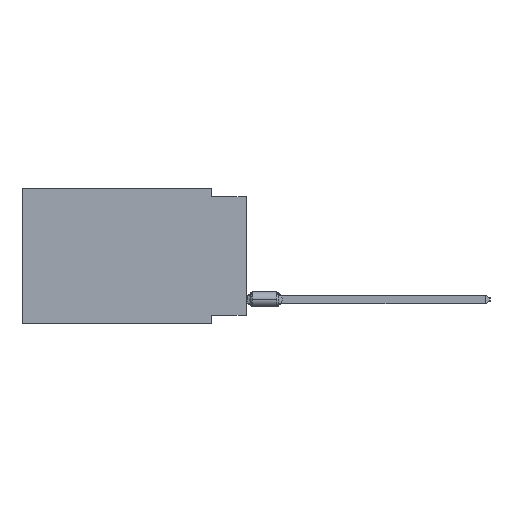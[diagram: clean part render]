
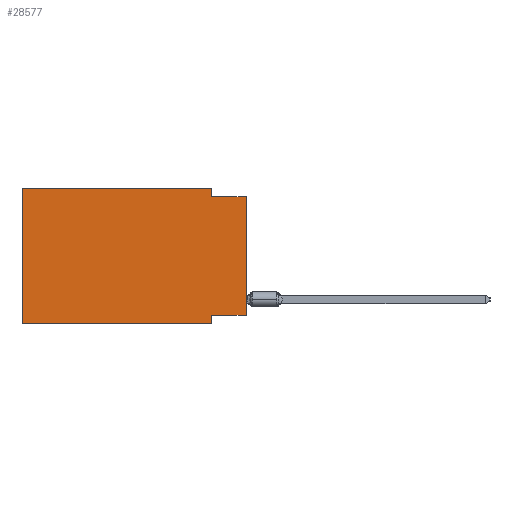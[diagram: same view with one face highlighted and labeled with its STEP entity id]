
A CAD part, left-side view. The second image highlights one B-rep face of the part: STEP entity #28577.
In plain terms, the highlighted planar face has unit normal (-1, 0, 0).
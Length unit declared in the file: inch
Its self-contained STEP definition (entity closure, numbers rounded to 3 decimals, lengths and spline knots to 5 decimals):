
#145 = VECTOR ( 'NONE', #30074, 39.37008 ) ;
#1103 = CARTESIAN_POINT ( 'NONE',  ( 0., 0., -0.365 ) ) ;
#1312 = DIRECTION ( 'NONE',  ( 0., -1., 0. ) ) ;
#1321 = ORIENTED_EDGE ( 'NONE', *, *, #29174, .T. ) ;
#2179 = CARTESIAN_POINT ( 'NONE',  ( 0., 0.645, 0. ) ) ;
#2435 = LINE ( 'NONE', #18656, #37084 ) ;
#2468 = LINE ( 'NONE', #34897, #15779 ) ;
#3201 = ORIENTED_EDGE ( 'NONE', *, *, #27384, .F. ) ;
#3221 = EDGE_CURVE ( 'NONE', #34792, #11804, #46527, .T. ) ;
#5310 = CARTESIAN_POINT ( 'NONE',  ( 0., 0.645, -0.39 ) ) ;
#5547 = CARTESIAN_POINT ( 'NONE',  ( 0., 0., -0.365 ) ) ;
#6477 = VECTOR ( 'NONE', #13910, 39.37008 ) ;
#7226 = DIRECTION ( 'NONE',  ( 0., 0., -1. ) ) ;
#8463 = ORIENTED_EDGE ( 'NONE', *, *, #50432, .F. ) ;
#8610 = VECTOR ( 'NONE', #34588, 39.37008 ) ;
#8622 = EDGE_CURVE ( 'NONE', #34792, #28995, #41442, .T. ) ;
#9359 = CARTESIAN_POINT ( 'NONE',  ( 0., 0.645, 0. ) ) ;
#11427 = CARTESIAN_POINT ( 'NONE',  ( 0., 0.1, 0. ) ) ;
#11472 = CARTESIAN_POINT ( 'NONE',  ( 0., 0., -0.025 ) ) ;
#11804 = VERTEX_POINT ( 'NONE', #32282 ) ;
#11856 = ORIENTED_EDGE ( 'NONE', *, *, #8622, .T. ) ;
#13594 = VERTEX_POINT ( 'NONE', #11427 ) ;
#13744 = VERTEX_POINT ( 'NONE', #33440 ) ;
#13910 = DIRECTION ( 'NONE',  ( 0., -1., 0. ) ) ;
#14241 = CARTESIAN_POINT ( 'NONE',  ( 0., 0.645, 0. ) ) ;
#14652 = EDGE_LOOP ( 'NONE', ( #1321, #3201, #19475, #15626, #17427, #11856, #8463, #35387 ) ) ;
#15626 = ORIENTED_EDGE ( 'NONE', *, *, #48692, .F. ) ;
#15779 = VECTOR ( 'NONE', #30926, 39.37008 ) ;
#16359 = VERTEX_POINT ( 'NONE', #1103 ) ;
#17427 = ORIENTED_EDGE ( 'NONE', *, *, #3221, .F. ) ;
#18045 = LINE ( 'NONE', #5547, #22637 ) ;
#18418 = LINE ( 'NONE', #22664, #6477 ) ;
#18656 = CARTESIAN_POINT ( 'NONE',  ( 0., 0.1, 0. ) ) ;
#19475 = ORIENTED_EDGE ( 'NONE', *, *, #33443, .F. ) ;
#21434 = VERTEX_POINT ( 'NONE', #30998 ) ;
#21688 = DIRECTION ( 'NONE',  ( 0., 0., -1. ) ) ;
#21935 = DIRECTION ( 'NONE',  ( 1., 0., 0. ) ) ;
#22637 = VECTOR ( 'NONE', #25992, 39.37008 ) ;
#22664 = CARTESIAN_POINT ( 'NONE',  ( 0., 0., -0.025 ) ) ;
#25992 = DIRECTION ( 'NONE',  ( 0., 1., 0. ) ) ;
#27384 = EDGE_CURVE ( 'NONE', #21434, #31861, #18418, .T. ) ;
#27953 = CARTESIAN_POINT ( 'NONE',  ( 0., 0.645, -0.39 ) ) ;
#28157 = EDGE_CURVE ( 'NONE', #16359, #13744, #18045, .T. ) ;
#28161 = CARTESIAN_POINT ( 'NONE',  ( 0., 0.1, -0.39 ) ) ;
#28577 = ADVANCED_FACE ( 'NONE', ( #49831 ), #41899, .F. ) ;
#28995 = VERTEX_POINT ( 'NONE', #38086 ) ;
#29174 = EDGE_CURVE ( 'NONE', #16359, #31861, #2468, .T. ) ;
#30074 = DIRECTION ( 'NONE',  ( 0., 0., 1. ) ) ;
#30926 = DIRECTION ( 'NONE',  ( 0., 0., 1. ) ) ;
#30998 = CARTESIAN_POINT ( 'NONE',  ( 0., 0.1, -0.025 ) ) ;
#31861 = VERTEX_POINT ( 'NONE', #11472 ) ;
#32282 = CARTESIAN_POINT ( 'NONE',  ( 0., 0.645, 0. ) ) ;
#33440 = CARTESIAN_POINT ( 'NONE',  ( 0., 0.1, -0.365 ) ) ;
#33443 = EDGE_CURVE ( 'NONE', #13594, #21434, #2435, .T. ) ;
#34588 = DIRECTION ( 'NONE',  ( 0., -1., 0. ) ) ;
#34792 = VERTEX_POINT ( 'NONE', #27953 ) ;
#34897 = CARTESIAN_POINT ( 'NONE',  ( 0., 0., 0. ) ) ;
#35387 = ORIENTED_EDGE ( 'NONE', *, *, #28157, .F. ) ;
#36122 = LINE ( 'NONE', #28161, #36595 ) ;
#36595 = VECTOR ( 'NONE', #44363, 39.37008 ) ;
#37084 = VECTOR ( 'NONE', #7226, 39.37008 ) ;
#38086 = CARTESIAN_POINT ( 'NONE',  ( 0., 0.1, -0.39 ) ) ;
#38591 = LINE ( 'NONE', #2179, #8610 ) ;
#41442 = LINE ( 'NONE', #5310, #50048 ) ;
#41899 = PLANE ( 'NONE',  #43760 ) ;
#43760 = AXIS2_PLACEMENT_3D ( 'NONE', #14241, #21935, #21688 ) ;
#44363 = DIRECTION ( 'NONE',  ( 0., 0., -1. ) ) ;
#46527 = LINE ( 'NONE', #9359, #145 ) ;
#48692 = EDGE_CURVE ( 'NONE', #11804, #13594, #38591, .T. ) ;
#49831 = FACE_OUTER_BOUND ( 'NONE', #14652, .T. ) ;
#50048 = VECTOR ( 'NONE', #1312, 39.37008 ) ;
#50432 = EDGE_CURVE ( 'NONE', #13744, #28995, #36122, .T. ) ;
